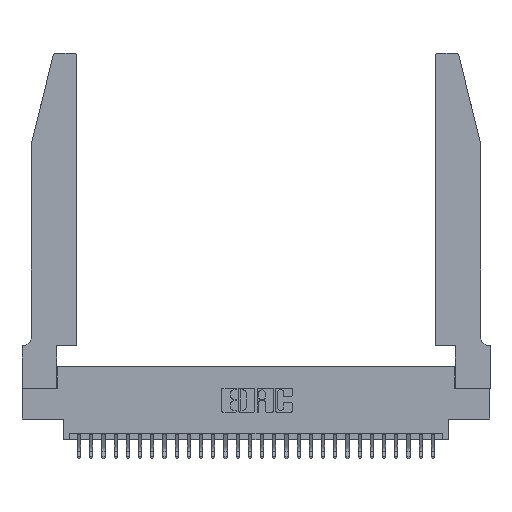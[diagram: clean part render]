
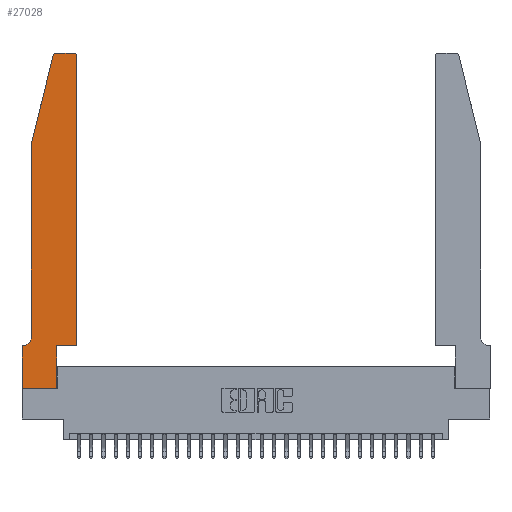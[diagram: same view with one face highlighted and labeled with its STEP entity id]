
A CAD part, top view. The second image highlights one B-rep face of the part: STEP entity #27028.
In plain terms, the highlighted planar face has unit normal (0, 0, 1).
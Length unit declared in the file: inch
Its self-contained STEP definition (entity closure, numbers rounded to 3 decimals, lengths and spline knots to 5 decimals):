
#470 = AXIS2_PLACEMENT_3D ( 'NONE', #2862, #19283, #5236 ) ;
#767 = CARTESIAN_POINT ( 'NONE',  ( 0.0755, 0.35, 0.37 ) ) ;
#1122 = ORIENTED_EDGE ( 'NONE', *, *, #18371, .T. ) ;
#1292 = VERTEX_POINT ( 'NONE', #19984 ) ;
#1419 = ORIENTED_EDGE ( 'NONE', *, *, #17662, .T. ) ;
#1441 = DIRECTION ( 'NONE',  ( 0., 0., 1. ) ) ;
#1694 = EDGE_CURVE ( 'NONE', #22830, #23792, #7187, .T. ) ;
#2040 = ORIENTED_EDGE ( 'NONE', *, *, #1694, .T. ) ;
#2408 = VECTOR ( 'NONE', #20610, 39.37008 ) ;
#2413 = ORIENTED_EDGE ( 'NONE', *, *, #10177, .T. ) ;
#2428 = DIRECTION ( 'NONE',  ( 0., 1., 0. ) ) ;
#2862 = CARTESIAN_POINT ( 'NONE',  ( 0.0055, 0.42, 0.37 ) ) ;
#3139 = DIRECTION ( 'NONE',  ( -1., 0., 0. ) ) ;
#3235 = EDGE_CURVE ( 'NONE', #11220, #23993, #27571, .T. ) ;
#3398 = AXIS2_PLACEMENT_3D ( 'NONE', #20173, #6148, #22496 ) ;
#4362 = ORIENTED_EDGE ( 'NONE', *, *, #6627, .T. ) ;
#4688 = CARTESIAN_POINT ( 'NONE',  ( 0.2865, 0.35, 0.37 ) ) ;
#5236 = DIRECTION ( 'NONE',  ( -1., 0., 0. ) ) ;
#5403 = CARTESIAN_POINT ( 'NONE',  ( 0., 0., 0.37 ) ) ;
#5709 = VERTEX_POINT ( 'NONE', #7530 ) ;
#6069 = CARTESIAN_POINT ( 'NONE',  ( 0.0755, 2., 0.37 ) ) ;
#6148 = DIRECTION ( 'NONE',  ( 0., 0., 1. ) ) ;
#6627 = EDGE_CURVE ( 'NONE', #1292, #22830, #9540, .T. ) ;
#7129 = DIRECTION ( 'NONE',  ( -0.239, -0.971, 0. ) ) ;
#7187 = LINE ( 'NONE', #5403, #18923 ) ;
#7416 = CIRCLE ( 'NONE', #24425, 0.03 ) ;
#7530 = CARTESIAN_POINT ( 'NONE',  ( 0.4205, 2.75, 0.37 ) ) ;
#7759 = CARTESIAN_POINT ( 'NONE',  ( 0.284, 2.75, 0.37 ) ) ;
#8149 = CIRCLE ( 'NONE', #3398, 0.03 ) ;
#8533 = CARTESIAN_POINT ( 'NONE',  ( 0.4505, 0.35, 0.37 ) ) ;
#8654 = CARTESIAN_POINT ( 'NONE',  ( 0.4505, 2.72, 0.37 ) ) ;
#8755 = DIRECTION ( 'NONE',  ( -1., 0., 0. ) ) ;
#8919 = VECTOR ( 'NONE', #13223, 39.37008 ) ;
#9256 = EDGE_LOOP ( 'NONE', ( #1122, #15410, #9853, #15237, #2413, #21538, #4362, #2040, #15840, #28344, #9617, #1419 ) ) ;
#9540 = LINE ( 'NONE', #29590, #21249 ) ;
#9617 = ORIENTED_EDGE ( 'NONE', *, *, #14191, .T. ) ;
#9853 = ORIENTED_EDGE ( 'NONE', *, *, #11307, .T. ) ;
#10177 = EDGE_CURVE ( 'NONE', #28025, #24584, #20646, .T. ) ;
#11078 = EDGE_CURVE ( 'NONE', #11997, #19860, #7416, .T. ) ;
#11220 = VERTEX_POINT ( 'NONE', #23318 ) ;
#11233 = LINE ( 'NONE', #767, #22978 ) ;
#11307 = EDGE_CURVE ( 'NONE', #19860, #25909, #26426, .T. ) ;
#11841 = CARTESIAN_POINT ( 'NONE',  ( 0.25487, 2.72718, 0.37 ) ) ;
#11997 = VERTEX_POINT ( 'NONE', #7759 ) ;
#12203 = AXIS2_PLACEMENT_3D ( 'NONE', #13138, #1441, #17875 ) ;
#12415 = LINE ( 'NONE', #4688, #24149 ) ;
#13040 = CARTESIAN_POINT ( 'NONE',  ( 0.284, 2.72, 0.37 ) ) ;
#13138 = CARTESIAN_POINT ( 'NONE',  ( 0., 0.35, 0.37 ) ) ;
#13223 = DIRECTION ( 'NONE',  ( 1., 0., 0. ) ) ;
#13547 = CARTESIAN_POINT ( 'NONE',  ( 0.0755, 2., 0.37 ) ) ;
#14121 = CARTESIAN_POINT ( 'NONE',  ( 0.2865, 0., 0.37 ) ) ;
#14191 = EDGE_CURVE ( 'NONE', #23993, #15194, #19320, .T. ) ;
#14440 = CARTESIAN_POINT ( 'NONE',  ( 0.0755, 0.42, 0.37 ) ) ;
#14685 = VECTOR ( 'NONE', #8755, 39.37008 ) ;
#15194 = VERTEX_POINT ( 'NONE', #8654 ) ;
#15237 = ORIENTED_EDGE ( 'NONE', *, *, #24752, .T. ) ;
#15410 = ORIENTED_EDGE ( 'NONE', *, *, #11078, .T. ) ;
#15694 = CARTESIAN_POINT ( 'NONE',  ( 0.2605, 2.75, 0.37 ) ) ;
#15811 = DIRECTION ( 'NONE',  ( 1., 0., 0. ) ) ;
#15840 = ORIENTED_EDGE ( 'NONE', *, *, #22482, .T. ) ;
#16435 = CARTESIAN_POINT ( 'NONE',  ( 0.0755, 2., 0.37 ) ) ;
#17557 = CARTESIAN_POINT ( 'NONE',  ( 0.0055, 0.35, 0.37 ) ) ;
#17662 = EDGE_CURVE ( 'NONE', #15194, #5709, #8149, .T. ) ;
#17875 = DIRECTION ( 'NONE',  ( 1., 0., 0. ) ) ;
#18371 = EDGE_CURVE ( 'NONE', #5709, #11997, #27121, .T. ) ;
#18580 = VECTOR ( 'NONE', #27364, 39.37008 ) ;
#18923 = VECTOR ( 'NONE', #26671, 39.37008 ) ;
#19283 = DIRECTION ( 'NONE',  ( 0., 0., -1. ) ) ;
#19320 = LINE ( 'NONE', #25013, #18580 ) ;
#19860 = VERTEX_POINT ( 'NONE', #11841 ) ;
#19984 = CARTESIAN_POINT ( 'NONE',  ( 0., 0.35, 0.37 ) ) ;
#20173 = CARTESIAN_POINT ( 'NONE',  ( 0.4205, 2.72, 0.37 ) ) ;
#20371 = DIRECTION ( 'NONE',  ( 0., -1., 0. ) ) ;
#20397 = LINE ( 'NONE', #13547, #2408 ) ;
#20610 = DIRECTION ( 'NONE',  ( 0., -1., 0. ) ) ;
#20646 = CIRCLE ( 'NONE', #470, 0.07 ) ;
#21249 = VECTOR ( 'NONE', #20371, 39.37008 ) ;
#21538 = ORIENTED_EDGE ( 'NONE', *, *, #26341, .T. ) ;
#22001 = CARTESIAN_POINT ( 'NONE',  ( 0.4505, 0.35, 0.37 ) ) ;
#22482 = EDGE_CURVE ( 'NONE', #23792, #11220, #12415, .T. ) ;
#22496 = DIRECTION ( 'NONE',  ( 1., 0., 0. ) ) ;
#22830 = VERTEX_POINT ( 'NONE', #22921 ) ;
#22921 = CARTESIAN_POINT ( 'NONE',  ( 0., 0., 0.37 ) ) ;
#22978 = VECTOR ( 'NONE', #3139, 39.37008 ) ;
#23318 = CARTESIAN_POINT ( 'NONE',  ( 0.2865, 0.35, 0.37 ) ) ;
#23792 = VERTEX_POINT ( 'NONE', #14121 ) ;
#23993 = VERTEX_POINT ( 'NONE', #22001 ) ;
#24149 = VECTOR ( 'NONE', #2428, 39.37008 ) ;
#24425 = AXIS2_PLACEMENT_3D ( 'NONE', #13040, #29363, #15811 ) ;
#24584 = VERTEX_POINT ( 'NONE', #17557 ) ;
#24752 = EDGE_CURVE ( 'NONE', #25909, #28025, #20397, .T. ) ;
#25013 = CARTESIAN_POINT ( 'NONE',  ( 0.4505, 0.35, 0.37 ) ) ;
#25687 = VECTOR ( 'NONE', #7129, 39.37008 ) ;
#25909 = VERTEX_POINT ( 'NONE', #6069 ) ;
#26341 = EDGE_CURVE ( 'NONE', #24584, #1292, #11233, .T. ) ;
#26426 = LINE ( 'NONE', #16435, #25687 ) ;
#26671 = DIRECTION ( 'NONE',  ( 1., 0., 0. ) ) ;
#27028 = ADVANCED_FACE ( 'NONE', ( #30173 ), #29454, .T. ) ;
#27121 = LINE ( 'NONE', #15694, #14685 ) ;
#27364 = DIRECTION ( 'NONE',  ( 0., 1., 0. ) ) ;
#27571 = LINE ( 'NONE', #8533, #8919 ) ;
#28025 = VERTEX_POINT ( 'NONE', #14440 ) ;
#28344 = ORIENTED_EDGE ( 'NONE', *, *, #3235, .T. ) ;
#29363 = DIRECTION ( 'NONE',  ( 0., 0., 1. ) ) ;
#29454 = PLANE ( 'NONE',  #12203 ) ;
#29590 = CARTESIAN_POINT ( 'NONE',  ( 0., 0., 0.37 ) ) ;
#30173 = FACE_OUTER_BOUND ( 'NONE', #9256, .T. ) ;
